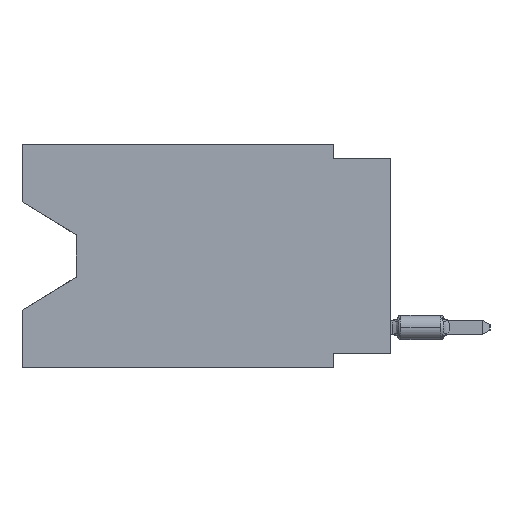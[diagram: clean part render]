
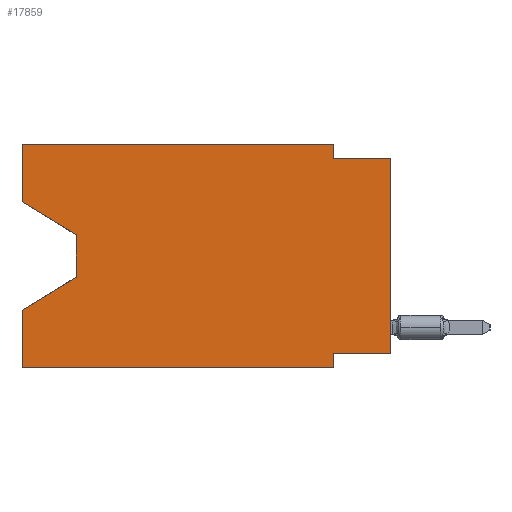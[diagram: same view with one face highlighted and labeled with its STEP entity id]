
A CAD part, left-side view. The second image highlights one B-rep face of the part: STEP entity #17859.
In plain terms, the highlighted planar face has unit normal (-1, 0, 0).
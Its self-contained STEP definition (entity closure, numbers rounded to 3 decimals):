
#221 = VERTEX_POINT ( 'NONE', #15765 ) ;
#551 = EDGE_CURVE ( 'NONE', #14568, #221, #22380, .T. ) ;
#737 = CARTESIAN_POINT ( 'NONE',  ( 0., 16.383, 0. ) ) ;
#797 = VERTEX_POINT ( 'NONE', #21134 ) ;
#1069 = LINE ( 'NONE', #17640, #25275 ) ;
#1245 = VECTOR ( 'NONE', #22249, 1000. ) ;
#2355 = EDGE_CURVE ( 'NONE', #6281, #14056, #25431, .T. ) ;
#2420 = VERTEX_POINT ( 'NONE', #22645 ) ;
#2469 = FACE_OUTER_BOUND ( 'NONE', #9876, .T. ) ;
#2568 = ORIENTED_EDGE ( 'NONE', *, *, #20655, .F. ) ;
#3363 = CARTESIAN_POINT ( 'NONE',  ( 0., 16.383, 0. ) ) ;
#3578 = EDGE_CURVE ( 'NONE', #29435, #14568, #20347, .T. ) ;
#3611 = ORIENTED_EDGE ( 'NONE', *, *, #2355, .F. ) ;
#3688 = ORIENTED_EDGE ( 'NONE', *, *, #551, .T. ) ;
#3891 = AXIS2_PLACEMENT_3D ( 'NONE', #737, #9592, #14842 ) ;
#4204 = VERTEX_POINT ( 'NONE', #20547 ) ;
#4331 = LINE ( 'NONE', #16098, #12185 ) ;
#4473 = CARTESIAN_POINT ( 'NONE',  ( 0., 16.383, 0. ) ) ;
#4550 = CARTESIAN_POINT ( 'NONE',  ( 0., 16.383, -2.546 ) ) ;
#4839 = VERTEX_POINT ( 'NONE', #13697 ) ;
#5235 = ORIENTED_EDGE ( 'NONE', *, *, #5632, .F. ) ;
#5238 = PLANE ( 'NONE',  #3891 ) ;
#5632 = EDGE_CURVE ( 'NONE', #29435, #4839, #17756, .T. ) ;
#5670 = CARTESIAN_POINT ( 'NONE',  ( 0., 13.97, -5.893 ) ) ;
#6043 = ORIENTED_EDGE ( 'NONE', *, *, #7786, .F. ) ;
#6281 = VERTEX_POINT ( 'NONE', #10332 ) ;
#6532 = EDGE_CURVE ( 'NONE', #20590, #4204, #18672, .T. ) ;
#6908 = ORIENTED_EDGE ( 'NONE', *, *, #3578, .T. ) ;
#6922 = CARTESIAN_POINT ( 'NONE',  ( 0., 0., -9.271 ) ) ;
#7786 = EDGE_CURVE ( 'NONE', #4839, #21655, #23670, .T. ) ;
#7852 = CARTESIAN_POINT ( 'NONE',  ( 0., 0., -0.635 ) ) ;
#7984 = DIRECTION ( 'NONE',  ( 0., 0., -1. ) ) ;
#8291 = CARTESIAN_POINT ( 'NONE',  ( 0., 13.97, -4.013 ) ) ;
#8817 = DIRECTION ( 'NONE',  ( 0., 0., -1. ) ) ;
#9192 = CARTESIAN_POINT ( 'NONE',  ( 0., 16.383, -9.906 ) ) ;
#9592 = DIRECTION ( 'NONE',  ( 1., 0., 0. ) ) ;
#9764 = VECTOR ( 'NONE', #24684, 1000. ) ;
#9876 = EDGE_LOOP ( 'NONE', ( #6908, #3688, #23608, #2568, #18195, #22530, #13684, #12135, #3611, #11220, #6043, #5235 ) ) ;
#10061 = VECTOR ( 'NONE', #16798, 1000. ) ;
#10332 = CARTESIAN_POINT ( 'NONE',  ( 0., 2.54, -0.635 ) ) ;
#10442 = VECTOR ( 'NONE', #20811, 1000. ) ;
#11220 = ORIENTED_EDGE ( 'NONE', *, *, #19916, .F. ) ;
#12135 = ORIENTED_EDGE ( 'NONE', *, *, #18007, .T. ) ;
#12185 = VECTOR ( 'NONE', #22901, 1000. ) ;
#12332 = CARTESIAN_POINT ( 'NONE',  ( 0., 16.383, -7.36 ) ) ;
#12981 = LINE ( 'NONE', #17773, #23677 ) ;
#13042 = DIRECTION ( 'NONE',  ( 0., -1., 0. ) ) ;
#13684 = ORIENTED_EDGE ( 'NONE', *, *, #6532, .F. ) ;
#13697 = CARTESIAN_POINT ( 'NONE',  ( 0., 16.383, 0. ) ) ;
#13920 = VECTOR ( 'NONE', #7984, 1000. ) ;
#14056 = VERTEX_POINT ( 'NONE', #7852 ) ;
#14568 = VERTEX_POINT ( 'NONE', #20493 ) ;
#14842 = DIRECTION ( 'NONE',  ( 0., 0., -1. ) ) ;
#15073 = CARTESIAN_POINT ( 'NONE',  ( 0., 2.54, 0. ) ) ;
#15450 = DIRECTION ( 'NONE',  ( 0., 0., 1. ) ) ;
#15765 = CARTESIAN_POINT ( 'NONE',  ( 0., 13.97, -5.893 ) ) ;
#16098 = CARTESIAN_POINT ( 'NONE',  ( 0., 16.383, 0. ) ) ;
#16798 = DIRECTION ( 'NONE',  ( 0., 1., 0. ) ) ;
#17640 = CARTESIAN_POINT ( 'NONE',  ( 0., 2.54, -9.906 ) ) ;
#17756 = LINE ( 'NONE', #3363, #1245 ) ;
#17773 = CARTESIAN_POINT ( 'NONE',  ( 0., 0., 0. ) ) ;
#17859 = ADVANCED_FACE ( 'NONE', ( #2469 ), #5238, .F. ) ;
#18007 = EDGE_CURVE ( 'NONE', #20590, #14056, #12981, .T. ) ;
#18195 = ORIENTED_EDGE ( 'NONE', *, *, #20046, .T. ) ;
#18672 = LINE ( 'NONE', #6922, #10061 ) ;
#18840 = CARTESIAN_POINT ( 'NONE',  ( 0., 16.383, -2.546 ) ) ;
#19385 = VERTEX_POINT ( 'NONE', #12332 ) ;
#19916 = EDGE_CURVE ( 'NONE', #21655, #6281, #29633, .T. ) ;
#20046 = EDGE_CURVE ( 'NONE', #2420, #797, #22660, .T. ) ;
#20347 = LINE ( 'NONE', #4550, #10442 ) ;
#20493 = CARTESIAN_POINT ( 'NONE',  ( 0., 13.97, -4.013 ) ) ;
#20547 = CARTESIAN_POINT ( 'NONE',  ( 0., 2.54, -9.271 ) ) ;
#20590 = VERTEX_POINT ( 'NONE', #26942 ) ;
#20655 = EDGE_CURVE ( 'NONE', #2420, #19385, #4331, .T. ) ;
#20811 = DIRECTION ( 'NONE',  ( 0., -0.855, -0.519 ) ) ;
#21134 = CARTESIAN_POINT ( 'NONE',  ( 0., 2.54, -9.906 ) ) ;
#21622 = VECTOR ( 'NONE', #27926, 1000. ) ;
#21655 = VERTEX_POINT ( 'NONE', #21867 ) ;
#21867 = CARTESIAN_POINT ( 'NONE',  ( 0., 2.54, 0. ) ) ;
#22249 = DIRECTION ( 'NONE',  ( 0., 0., 1. ) ) ;
#22380 = LINE ( 'NONE', #8291, #13920 ) ;
#22394 = DIRECTION ( 'NONE',  ( 0., 0.855, -0.519 ) ) ;
#22530 = ORIENTED_EDGE ( 'NONE', *, *, #24656, .F. ) ;
#22645 = CARTESIAN_POINT ( 'NONE',  ( 0., 16.383, -9.906 ) ) ;
#22660 = LINE ( 'NONE', #9192, #21622 ) ;
#22901 = DIRECTION ( 'NONE',  ( 0., 0., 1. ) ) ;
#22982 = VECTOR ( 'NONE', #22394, 1000. ) ;
#23608 = ORIENTED_EDGE ( 'NONE', *, *, #27671, .T. ) ;
#23670 = LINE ( 'NONE', #4473, #26931 ) ;
#23677 = VECTOR ( 'NONE', #15450, 1000. ) ;
#24656 = EDGE_CURVE ( 'NONE', #4204, #797, #1069, .T. ) ;
#24684 = DIRECTION ( 'NONE',  ( 0., 0., -1. ) ) ;
#24731 = LINE ( 'NONE', #5670, #22982 ) ;
#25119 = CARTESIAN_POINT ( 'NONE',  ( 0., 0., -0.635 ) ) ;
#25275 = VECTOR ( 'NONE', #8817, 1000. ) ;
#25431 = LINE ( 'NONE', #25119, #30228 ) ;
#26127 = DIRECTION ( 'NONE',  ( 0., -1., 0. ) ) ;
#26931 = VECTOR ( 'NONE', #26127, 1000. ) ;
#26942 = CARTESIAN_POINT ( 'NONE',  ( 0., 0., -9.271 ) ) ;
#27671 = EDGE_CURVE ( 'NONE', #221, #19385, #24731, .T. ) ;
#27926 = DIRECTION ( 'NONE',  ( 0., -1., 0. ) ) ;
#29435 = VERTEX_POINT ( 'NONE', #18840 ) ;
#29633 = LINE ( 'NONE', #15073, #9764 ) ;
#30228 = VECTOR ( 'NONE', #13042, 1000. ) ;
